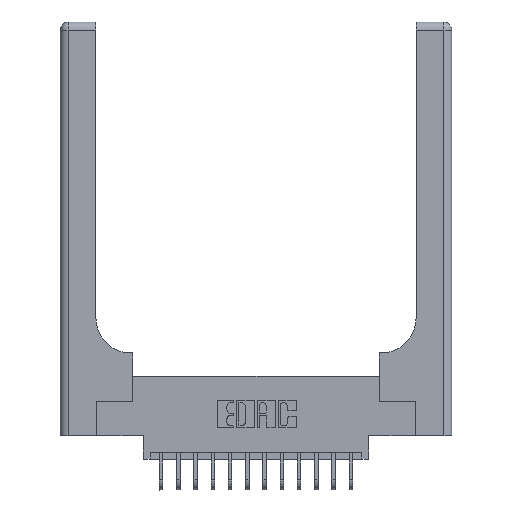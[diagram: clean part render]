
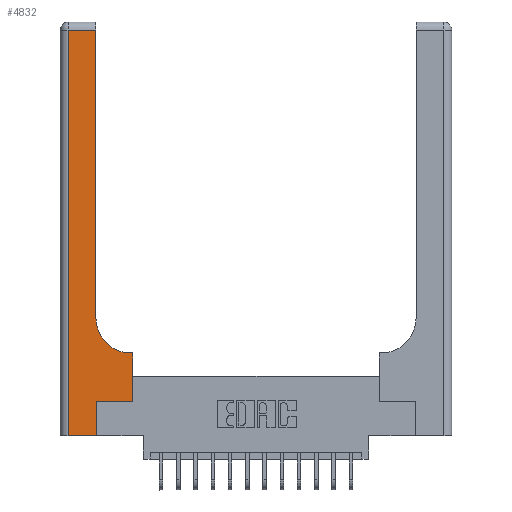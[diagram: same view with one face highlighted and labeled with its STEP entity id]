
A CAD part, top view. The second image highlights one B-rep face of the part: STEP entity #4832.
In plain terms, the highlighted planar face has unit normal (0, 0, 1).
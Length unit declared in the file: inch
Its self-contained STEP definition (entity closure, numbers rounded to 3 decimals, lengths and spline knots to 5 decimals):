
#1010 = ORIENTED_EDGE ( 'NONE', *, *, #4116, .T. ) ;
#1033 = DIRECTION ( 'NONE',  ( -1., 0., 0. ) ) ;
#1359 = CARTESIAN_POINT ( 'NONE',  ( 0.51, 0.85, 0.37 ) ) ;
#1435 = CIRCLE ( 'NONE', #7796, 0.25 ) ;
#1947 = ORIENTED_EDGE ( 'NONE', *, *, #15880, .T. ) ;
#2342 = CARTESIAN_POINT ( 'NONE',  ( 0.26, 0.85, 0.37 ) ) ;
#2606 = CARTESIAN_POINT ( 'NONE',  ( 0.265, 0.25, 0.37 ) ) ;
#2912 = CARTESIAN_POINT ( 'NONE',  ( 0., 2.94, 0.37 ) ) ;
#3165 = VERTEX_POINT ( 'NONE', #7451 ) ;
#3869 = EDGE_LOOP ( 'NONE', ( #11325, #6063, #1947, #16251, #9610, #16358, #1010, #11195, #8959 ) ) ;
#3924 = CARTESIAN_POINT ( 'NONE',  ( 0.26, 2.94, 0.37 ) ) ;
#3944 = VERTEX_POINT ( 'NONE', #2342 ) ;
#3960 = DIRECTION ( 'NONE',  ( 0., 1., 0. ) ) ;
#4023 = LINE ( 'NONE', #5484, #15205 ) ;
#4069 = PLANE ( 'NONE',  #12185 ) ;
#4116 = EDGE_CURVE ( 'NONE', #16534, #14544, #4774, .T. ) ;
#4354 = DIRECTION ( 'NONE',  ( -1., 0., 0. ) ) ;
#4774 = LINE ( 'NONE', #6382, #7940 ) ;
#4832 = ADVANCED_FACE ( 'NONE', ( #11587 ), #4069, .F. ) ;
#5107 = VERTEX_POINT ( 'NONE', #13634 ) ;
#5484 = CARTESIAN_POINT ( 'NONE',  ( 0.06, 3., 0.37 ) ) ;
#5725 = DIRECTION ( 'NONE',  ( -1., 0., 0. ) ) ;
#5727 = CARTESIAN_POINT ( 'NONE',  ( 0.265, 0., 0.37 ) ) ;
#6063 = ORIENTED_EDGE ( 'NONE', *, *, #11103, .T. ) ;
#6382 = CARTESIAN_POINT ( 'NONE',  ( 0.528, 0.25, 0.37 ) ) ;
#6406 = VECTOR ( 'NONE', #3960, 39.37008 ) ;
#7084 = EDGE_CURVE ( 'NONE', #14544, #12571, #16143, .T. ) ;
#7451 = CARTESIAN_POINT ( 'NONE',  ( 0.06, 0., 0.37 ) ) ;
#7622 = CARTESIAN_POINT ( 'NONE',  ( 0.26, 3., 0.37 ) ) ;
#7796 = AXIS2_PLACEMENT_3D ( 'NONE', #1359, #13412, #19329 ) ;
#7928 = VECTOR ( 'NONE', #1033, 39.37008 ) ;
#7940 = VECTOR ( 'NONE', #9563, 39.37008 ) ;
#8614 = VECTOR ( 'NONE', #18452, 39.37008 ) ;
#8907 = CARTESIAN_POINT ( 'NONE',  ( 0.265, 0.25, 0.37 ) ) ;
#8951 = EDGE_CURVE ( 'NONE', #13763, #16534, #11411, .T. ) ;
#8959 = ORIENTED_EDGE ( 'NONE', *, *, #13767, .T. ) ;
#9199 = LINE ( 'NONE', #12511, #8614 ) ;
#9444 = LINE ( 'NONE', #7622, #6406 ) ;
#9563 = DIRECTION ( 'NONE',  ( 0., 1., 0. ) ) ;
#9610 = ORIENTED_EDGE ( 'NONE', *, *, #9774, .T. ) ;
#9774 = EDGE_CURVE ( 'NONE', #12064, #13763, #13474, .T. ) ;
#10156 = CARTESIAN_POINT ( 'NONE',  ( 0., 3., 0.37 ) ) ;
#10453 = LINE ( 'NONE', #2912, #7928 ) ;
#10533 = DIRECTION ( 'NONE',  ( 0., 1., 0. ) ) ;
#11103 = EDGE_CURVE ( 'NONE', #18473, #5107, #10453, .T. ) ;
#11195 = ORIENTED_EDGE ( 'NONE', *, *, #7084, .T. ) ;
#11325 = ORIENTED_EDGE ( 'NONE', *, *, #13557, .T. ) ;
#11411 = LINE ( 'NONE', #2606, #18703 ) ;
#11587 = FACE_OUTER_BOUND ( 'NONE', #3869, .T. ) ;
#12064 = VERTEX_POINT ( 'NONE', #5727 ) ;
#12185 = AXIS2_PLACEMENT_3D ( 'NONE', #10156, #16062, #4354 ) ;
#12298 = EDGE_CURVE ( 'NONE', #3165, #12064, #9199, .T. ) ;
#12511 = CARTESIAN_POINT ( 'NONE',  ( 0., 0., 0.37 ) ) ;
#12571 = VERTEX_POINT ( 'NONE', #14693 ) ;
#12733 = CARTESIAN_POINT ( 'NONE',  ( 0.528, 0.25, 0.37 ) ) ;
#13412 = DIRECTION ( 'NONE',  ( 0., 0., -1. ) ) ;
#13474 = LINE ( 'NONE', #13566, #14714 ) ;
#13557 = EDGE_CURVE ( 'NONE', #3944, #18473, #9444, .T. ) ;
#13566 = CARTESIAN_POINT ( 'NONE',  ( 0.265, 0., 0.37 ) ) ;
#13634 = CARTESIAN_POINT ( 'NONE',  ( 0.06, 2.94, 0.37 ) ) ;
#13763 = VERTEX_POINT ( 'NONE', #8907 ) ;
#13767 = EDGE_CURVE ( 'NONE', #12571, #3944, #1435, .T. ) ;
#14244 = CARTESIAN_POINT ( 'NONE',  ( 0.528, 0.6, 0.37 ) ) ;
#14544 = VERTEX_POINT ( 'NONE', #14244 ) ;
#14691 = CARTESIAN_POINT ( 'NONE',  ( 0.26, 0.6, 0.37 ) ) ;
#14693 = CARTESIAN_POINT ( 'NONE',  ( 0.51, 0.6, 0.37 ) ) ;
#14714 = VECTOR ( 'NONE', #10533, 39.37008 ) ;
#15205 = VECTOR ( 'NONE', #18939, 39.37008 ) ;
#15880 = EDGE_CURVE ( 'NONE', #5107, #3165, #4023, .T. ) ;
#16000 = VECTOR ( 'NONE', #5725, 39.37008 ) ;
#16062 = DIRECTION ( 'NONE',  ( 0., 0., -1. ) ) ;
#16143 = LINE ( 'NONE', #14691, #16000 ) ;
#16251 = ORIENTED_EDGE ( 'NONE', *, *, #12298, .T. ) ;
#16358 = ORIENTED_EDGE ( 'NONE', *, *, #8951, .T. ) ;
#16534 = VERTEX_POINT ( 'NONE', #12733 ) ;
#17738 = DIRECTION ( 'NONE',  ( 1., 0., 0. ) ) ;
#18452 = DIRECTION ( 'NONE',  ( 1., 0., 0. ) ) ;
#18473 = VERTEX_POINT ( 'NONE', #3924 ) ;
#18703 = VECTOR ( 'NONE', #17738, 39.37008 ) ;
#18939 = DIRECTION ( 'NONE',  ( 0., -1., 0. ) ) ;
#19329 = DIRECTION ( 'NONE',  ( 1., 0., 0. ) ) ;
